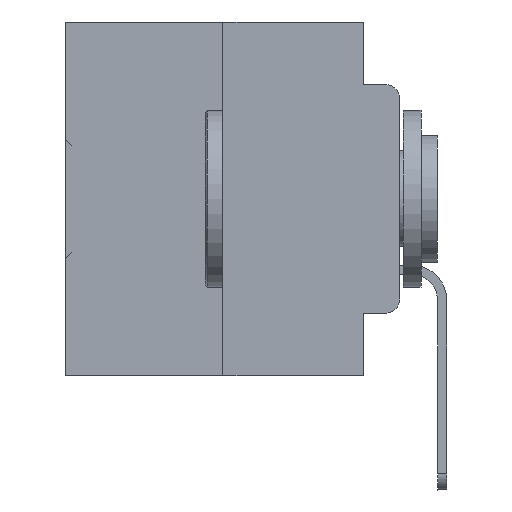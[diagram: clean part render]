
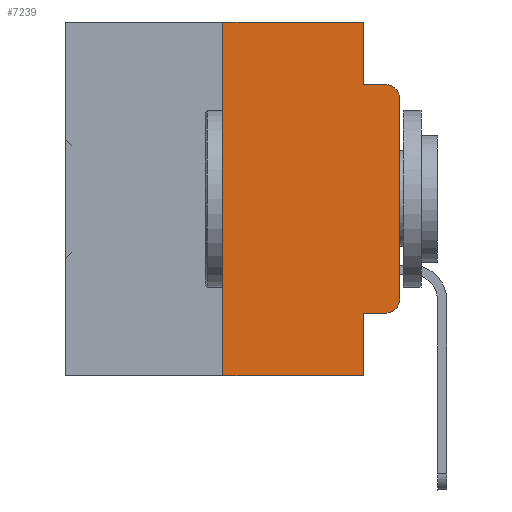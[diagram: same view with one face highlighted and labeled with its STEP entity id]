
A CAD part, left-side view. The second image highlights one B-rep face of the part: STEP entity #7239.
In plain terms, the highlighted planar face has unit normal (-1, 0, 0).
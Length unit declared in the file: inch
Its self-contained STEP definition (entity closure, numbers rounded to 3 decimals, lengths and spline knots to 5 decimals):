
#530 = EDGE_CURVE ( 'NONE', #8342, #32322, #20928, .T. ) ;
#577 = ORIENTED_EDGE ( 'NONE', *, *, #31778, .F. ) ;
#844 = VECTOR ( 'NONE', #31141, 39.37008 ) ;
#1027 = ORIENTED_EDGE ( 'NONE', *, *, #10748, .F. ) ;
#1238 = VECTOR ( 'NONE', #14745, 39.37008 ) ;
#1699 = ORIENTED_EDGE ( 'NONE', *, *, #3418, .F. ) ;
#1717 = DIRECTION ( 'NONE',  ( -1., 0., 0. ) ) ;
#2436 = VERTEX_POINT ( 'NONE', #31022 ) ;
#2909 = EDGE_CURVE ( 'NONE', #23501, #26684, #30982, .T. ) ;
#3093 = LINE ( 'NONE', #14319, #31540 ) ;
#3418 = EDGE_CURVE ( 'NONE', #29061, #8342, #3093, .T. ) ;
#3436 = FACE_OUTER_BOUND ( 'NONE', #6968, .T. ) ;
#5009 = DIRECTION ( 'NONE',  ( 0., 0., -1. ) ) ;
#6049 = CARTESIAN_POINT ( 'NONE',  ( 0., 0.25, 0. ) ) ;
#6968 = EDGE_LOOP ( 'NONE', ( #9560, #36443, #25757, #1699, #577, #8156, #22934, #1027, #25671, #20308 ) ) ;
#7239 = ADVANCED_FACE ( 'NONE', ( #3436 ), #14668, .F. ) ;
#7318 = DIRECTION ( 'NONE',  ( 0., -1., 0. ) ) ;
#7653 = DIRECTION ( 'NONE',  ( 0., 0., -1. ) ) ;
#7734 = CARTESIAN_POINT ( 'NONE',  ( 0., 0.051, 0. ) ) ;
#8156 = ORIENTED_EDGE ( 'NONE', *, *, #20817, .F. ) ;
#8229 = AXIS2_PLACEMENT_3D ( 'NONE', #10724, #1717, #5009 ) ;
#8244 = DIRECTION ( 'NONE',  ( 0., -1., 0. ) ) ;
#8342 = VERTEX_POINT ( 'NONE', #28698 ) ;
#9560 = ORIENTED_EDGE ( 'NONE', *, *, #2909, .T. ) ;
#9724 = CIRCLE ( 'NONE', #22102, 0.02 ) ;
#10520 = VERTEX_POINT ( 'NONE', #25466 ) ;
#10724 = CARTESIAN_POINT ( 'NONE',  ( 0., 0.02, -0.1085 ) ) ;
#10748 = EDGE_CURVE ( 'NONE', #34208, #10520, #30056, .T. ) ;
#10804 = CARTESIAN_POINT ( 'NONE',  ( 0., 0.473, 0. ) ) ;
#11597 = DIRECTION ( 'NONE',  ( 0., 0., 1. ) ) ;
#12781 = CARTESIAN_POINT ( 'NONE',  ( 0., 0.051, -0.4115 ) ) ;
#14319 = CARTESIAN_POINT ( 'NONE',  ( 0., 0.051, 0. ) ) ;
#14346 = LINE ( 'NONE', #6049, #844 ) ;
#14668 = PLANE ( 'NONE',  #26377 ) ;
#14745 = DIRECTION ( 'NONE',  ( 0., -1., 0. ) ) ;
#15747 = CARTESIAN_POINT ( 'NONE',  ( 0., 0.051, -0.0885 ) ) ;
#16181 = CARTESIAN_POINT ( 'NONE',  ( 0., 0.473, -0.5 ) ) ;
#16964 = CARTESIAN_POINT ( 'NONE',  ( 0., 0.051, -0.4115 ) ) ;
#17096 = VECTOR ( 'NONE', #32821, 39.37008 ) ;
#20308 = ORIENTED_EDGE ( 'NONE', *, *, #21536, .T. ) ;
#20558 = VERTEX_POINT ( 'NONE', #31920 ) ;
#20817 = EDGE_CURVE ( 'NONE', #20558, #30192, #14346, .T. ) ;
#20928 = LINE ( 'NONE', #15747, #29474 ) ;
#21536 = EDGE_CURVE ( 'NONE', #2436, #23501, #9724, .T. ) ;
#22102 = AXIS2_PLACEMENT_3D ( 'NONE', #22729, #22545, #31038 ) ;
#22545 = DIRECTION ( 'NONE',  ( -1., 0., 0. ) ) ;
#22729 = CARTESIAN_POINT ( 'NONE',  ( 0., 0.02, -0.3915 ) ) ;
#22934 = ORIENTED_EDGE ( 'NONE', *, *, #27930, .T. ) ;
#23087 = EDGE_CURVE ( 'NONE', #26684, #32322, #34133, .T. ) ;
#23501 = VERTEX_POINT ( 'NONE', #32818 ) ;
#24244 = CARTESIAN_POINT ( 'NONE',  ( 0., 0.02, -0.0885 ) ) ;
#25466 = CARTESIAN_POINT ( 'NONE',  ( 0., 0.051, -0.5 ) ) ;
#25671 = ORIENTED_EDGE ( 'NONE', *, *, #31171, .T. ) ;
#25757 = ORIENTED_EDGE ( 'NONE', *, *, #530, .F. ) ;
#26377 = AXIS2_PLACEMENT_3D ( 'NONE', #31655, #27394, #7653 ) ;
#26684 = VERTEX_POINT ( 'NONE', #30389 ) ;
#27394 = DIRECTION ( 'NONE',  ( 1., 0., 0. ) ) ;
#27642 = CARTESIAN_POINT ( 'NONE',  ( 0., 0.25, 0. ) ) ;
#27930 = EDGE_CURVE ( 'NONE', #20558, #10520, #30393, .T. ) ;
#28550 = VECTOR ( 'NONE', #11597, 39.37008 ) ;
#28698 = CARTESIAN_POINT ( 'NONE',  ( 0., 0.051, -0.0885 ) ) ;
#29061 = VERTEX_POINT ( 'NONE', #30216 ) ;
#29474 = VECTOR ( 'NONE', #32543, 39.37008 ) ;
#29640 = LINE ( 'NONE', #10804, #34259 ) ;
#30056 = LINE ( 'NONE', #7734, #17096 ) ;
#30192 = VERTEX_POINT ( 'NONE', #27642 ) ;
#30216 = CARTESIAN_POINT ( 'NONE',  ( 0., 0.051, 0. ) ) ;
#30389 = CARTESIAN_POINT ( 'NONE',  ( 0., 0., -0.1085 ) ) ;
#30393 = LINE ( 'NONE', #16181, #34925 ) ;
#30982 = LINE ( 'NONE', #33924, #28550 ) ;
#31022 = CARTESIAN_POINT ( 'NONE',  ( 0., 0.02, -0.4115 ) ) ;
#31038 = DIRECTION ( 'NONE',  ( 0., 0., -1. ) ) ;
#31141 = DIRECTION ( 'NONE',  ( 0., 0., 1. ) ) ;
#31171 = EDGE_CURVE ( 'NONE', #34208, #2436, #34304, .T. ) ;
#31540 = VECTOR ( 'NONE', #33159, 39.37008 ) ;
#31655 = CARTESIAN_POINT ( 'NONE',  ( 0., 0.473, 0. ) ) ;
#31778 = EDGE_CURVE ( 'NONE', #30192, #29061, #29640, .T. ) ;
#31920 = CARTESIAN_POINT ( 'NONE',  ( 0., 0.25, -0.5 ) ) ;
#32322 = VERTEX_POINT ( 'NONE', #24244 ) ;
#32543 = DIRECTION ( 'NONE',  ( 0., -1., 0. ) ) ;
#32818 = CARTESIAN_POINT ( 'NONE',  ( 0., 0., -0.3915 ) ) ;
#32821 = DIRECTION ( 'NONE',  ( 0., 0., -1. ) ) ;
#33159 = DIRECTION ( 'NONE',  ( 0., 0., -1. ) ) ;
#33924 = CARTESIAN_POINT ( 'NONE',  ( 0., 0., 0. ) ) ;
#34133 = CIRCLE ( 'NONE', #8229, 0.02 ) ;
#34208 = VERTEX_POINT ( 'NONE', #12781 ) ;
#34259 = VECTOR ( 'NONE', #7318, 39.37008 ) ;
#34304 = LINE ( 'NONE', #16964, #1238 ) ;
#34925 = VECTOR ( 'NONE', #8244, 39.37008 ) ;
#36443 = ORIENTED_EDGE ( 'NONE', *, *, #23087, .T. ) ;
